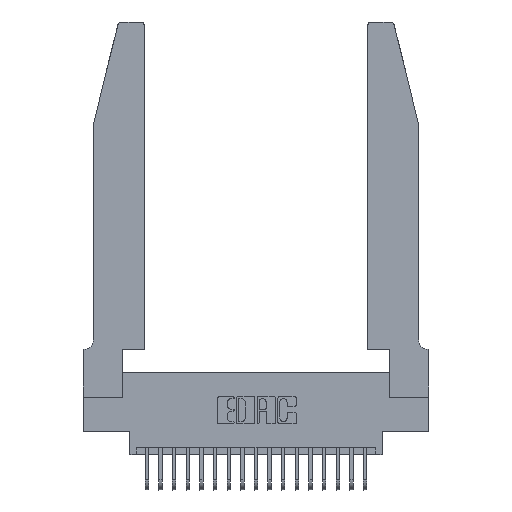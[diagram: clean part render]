
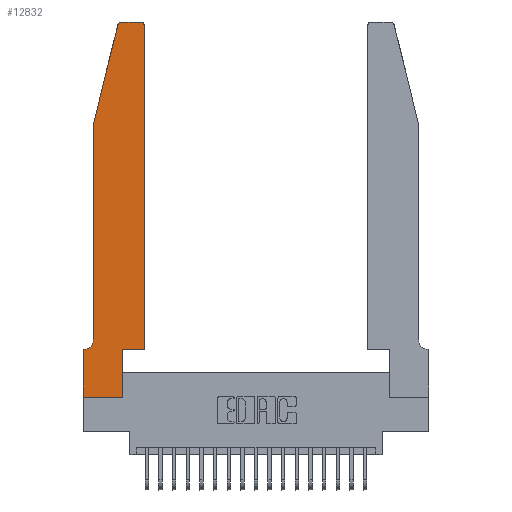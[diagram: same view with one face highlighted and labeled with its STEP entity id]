
A CAD part, top view. The second image highlights one B-rep face of the part: STEP entity #12832.
In plain terms, the highlighted planar face has unit normal (0, 0, 1).
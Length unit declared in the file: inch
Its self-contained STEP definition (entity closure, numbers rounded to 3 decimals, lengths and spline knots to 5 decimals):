
#241 = CARTESIAN_POINT ( 'NONE',  ( 0.2865, 0.35, 0.37 ) ) ;
#877 = EDGE_CURVE ( 'NONE', #9684, #13291, #17296, .T. ) ;
#950 = CARTESIAN_POINT ( 'NONE',  ( 0.4505, 0.35, 0.37 ) ) ;
#2104 = EDGE_CURVE ( 'NONE', #16932, #18440, #22708, .T. ) ;
#2256 = VECTOR ( 'NONE', #17035, 39.37008 ) ;
#2323 = CARTESIAN_POINT ( 'NONE',  ( 0., 0.35, 0.37 ) ) ;
#2464 = CARTESIAN_POINT ( 'NONE',  ( 0.0755, 2., 0.37 ) ) ;
#2515 = CARTESIAN_POINT ( 'NONE',  ( 0.0055, 0.42, 0.37 ) ) ;
#2593 = VERTEX_POINT ( 'NONE', #18004 ) ;
#2752 = AXIS2_PLACEMENT_3D ( 'NONE', #13253, #15020, #4253 ) ;
#3676 = CARTESIAN_POINT ( 'NONE',  ( 0.284, 2.72, 0.37 ) ) ;
#3970 = VERTEX_POINT ( 'NONE', #6643 ) ;
#4253 = DIRECTION ( 'NONE',  ( 1., 0., 0. ) ) ;
#4393 = DIRECTION ( 'NONE',  ( -1., 0., 0. ) ) ;
#4984 = ORIENTED_EDGE ( 'NONE', *, *, #7084, .T. ) ;
#5078 = VERTEX_POINT ( 'NONE', #16766 ) ;
#5187 = CARTESIAN_POINT ( 'NONE',  ( 0.2865, 0., 0.37 ) ) ;
#5199 = VECTOR ( 'NONE', #22372, 39.37008 ) ;
#5392 = CARTESIAN_POINT ( 'NONE',  ( 0.284, 2.75, 0.37 ) ) ;
#5557 = DIRECTION ( 'NONE',  ( 1., 0., 0. ) ) ;
#5711 = EDGE_CURVE ( 'NONE', #18440, #8548, #11969, .T. ) ;
#5781 = LINE ( 'NONE', #20601, #5199 ) ;
#6074 = ORIENTED_EDGE ( 'NONE', *, *, #11623, .T. ) ;
#6567 = VECTOR ( 'NONE', #8561, 39.37008 ) ;
#6643 = CARTESIAN_POINT ( 'NONE',  ( 0.4205, 2.75, 0.37 ) ) ;
#6813 = LINE ( 'NONE', #22697, #11026 ) ;
#6990 = ORIENTED_EDGE ( 'NONE', *, *, #877, .T. ) ;
#7084 = EDGE_CURVE ( 'NONE', #2593, #22466, #12456, .T. ) ;
#7121 = EDGE_CURVE ( 'NONE', #3970, #15149, #11331, .T. ) ;
#7130 = DIRECTION ( 'NONE',  ( 0., 1., 0. ) ) ;
#7306 = DIRECTION ( 'NONE',  ( -1., 0., 0. ) ) ;
#7678 = ORIENTED_EDGE ( 'NONE', *, *, #2104, .T. ) ;
#7838 = EDGE_CURVE ( 'NONE', #16422, #2593, #6813, .T. ) ;
#8370 = CARTESIAN_POINT ( 'NONE',  ( 0.0755, 0.35, 0.37 ) ) ;
#8452 = CARTESIAN_POINT ( 'NONE',  ( 0.4205, 2.72, 0.37 ) ) ;
#8548 = VERTEX_POINT ( 'NONE', #23055 ) ;
#8561 = DIRECTION ( 'NONE',  ( -1., 0., 0. ) ) ;
#8899 = ORIENTED_EDGE ( 'NONE', *, *, #13413, .T. ) ;
#8993 = AXIS2_PLACEMENT_3D ( 'NONE', #3676, #16250, #5557 ) ;
#9684 = VERTEX_POINT ( 'NONE', #2464 ) ;
#9938 = CARTESIAN_POINT ( 'NONE',  ( 0., 0., 0.37 ) ) ;
#10258 = DIRECTION ( 'NONE',  ( 1., 0., 0. ) ) ;
#10673 = CARTESIAN_POINT ( 'NONE',  ( 0.2865, 0.35, 0.37 ) ) ;
#10739 = DIRECTION ( 'NONE',  ( 0., -1., 0. ) ) ;
#11026 = VECTOR ( 'NONE', #13981, 39.37008 ) ;
#11293 = DIRECTION ( 'NONE',  ( 1., 0., 0. ) ) ;
#11321 = CARTESIAN_POINT ( 'NONE',  ( 0.0755, 2., 0.37 ) ) ;
#11331 = LINE ( 'NONE', #13852, #6567 ) ;
#11623 = EDGE_CURVE ( 'NONE', #5078, #9684, #5781, .T. ) ;
#11921 = DIRECTION ( 'NONE',  ( 0., 1., 0. ) ) ;
#11969 = LINE ( 'NONE', #9938, #2256 ) ;
#12070 = EDGE_CURVE ( 'NONE', #19820, #16422, #15271, .T. ) ;
#12185 = LINE ( 'NONE', #20187, #16854 ) ;
#12456 = LINE ( 'NONE', #950, #12991 ) ;
#12832 = ADVANCED_FACE ( 'NONE', ( #22622 ), #21972, .T. ) ;
#12991 = VECTOR ( 'NONE', #11921, 39.37008 ) ;
#13253 = CARTESIAN_POINT ( 'NONE',  ( 0., 0.35, 0.37 ) ) ;
#13291 = VERTEX_POINT ( 'NONE', #18077 ) ;
#13413 = EDGE_CURVE ( 'NONE', #8548, #19820, #12185, .T. ) ;
#13558 = EDGE_LOOP ( 'NONE', ( #17201, #16287, #6074, #6990, #14832, #7678, #20823, #8899, #17856, #15380, #4984, #17040 ) ) ;
#13852 = CARTESIAN_POINT ( 'NONE',  ( 0.2605, 2.75, 0.37 ) ) ;
#13981 = DIRECTION ( 'NONE',  ( 1., 0., 0. ) ) ;
#14418 = CARTESIAN_POINT ( 'NONE',  ( 0.0055, 0.35, 0.37 ) ) ;
#14725 = VECTOR ( 'NONE', #7130, 39.37008 ) ;
#14832 = ORIENTED_EDGE ( 'NONE', *, *, #17916, .T. ) ;
#15020 = DIRECTION ( 'NONE',  ( 0., 0., 1. ) ) ;
#15149 = VERTEX_POINT ( 'NONE', #5392 ) ;
#15150 = DIRECTION ( 'NONE',  ( 0., 0., -1. ) ) ;
#15271 = LINE ( 'NONE', #10673, #14725 ) ;
#15380 = ORIENTED_EDGE ( 'NONE', *, *, #7838, .T. ) ;
#15941 = CIRCLE ( 'NONE', #17163, 0.03 ) ;
#16250 = DIRECTION ( 'NONE',  ( 0., 0., 1. ) ) ;
#16287 = ORIENTED_EDGE ( 'NONE', *, *, #22155, .T. ) ;
#16422 = VERTEX_POINT ( 'NONE', #241 ) ;
#16766 = CARTESIAN_POINT ( 'NONE',  ( 0.25487, 2.72718, 0.37 ) ) ;
#16799 = CIRCLE ( 'NONE', #16855, 0.07 ) ;
#16854 = VECTOR ( 'NONE', #11293, 39.37008 ) ;
#16855 = AXIS2_PLACEMENT_3D ( 'NONE', #2515, #15150, #4393 ) ;
#16932 = VERTEX_POINT ( 'NONE', #14418 ) ;
#17035 = DIRECTION ( 'NONE',  ( 0., -1., 0. ) ) ;
#17040 = ORIENTED_EDGE ( 'NONE', *, *, #18639, .T. ) ;
#17163 = AXIS2_PLACEMENT_3D ( 'NONE', #8452, #20774, #10258 ) ;
#17201 = ORIENTED_EDGE ( 'NONE', *, *, #7121, .T. ) ;
#17296 = LINE ( 'NONE', #11321, #22483 ) ;
#17515 = VECTOR ( 'NONE', #7306, 39.37008 ) ;
#17856 = ORIENTED_EDGE ( 'NONE', *, *, #12070, .T. ) ;
#17916 = EDGE_CURVE ( 'NONE', #13291, #16932, #16799, .T. ) ;
#18004 = CARTESIAN_POINT ( 'NONE',  ( 0.4505, 0.35, 0.37 ) ) ;
#18077 = CARTESIAN_POINT ( 'NONE',  ( 0.0755, 0.42, 0.37 ) ) ;
#18440 = VERTEX_POINT ( 'NONE', #2323 ) ;
#18639 = EDGE_CURVE ( 'NONE', #22466, #3970, #15941, .T. ) ;
#19820 = VERTEX_POINT ( 'NONE', #5187 ) ;
#20018 = CIRCLE ( 'NONE', #8993, 0.03 ) ;
#20187 = CARTESIAN_POINT ( 'NONE',  ( 0., 0., 0.37 ) ) ;
#20502 = CARTESIAN_POINT ( 'NONE',  ( 0.4505, 2.72, 0.37 ) ) ;
#20601 = CARTESIAN_POINT ( 'NONE',  ( 0.0755, 2., 0.37 ) ) ;
#20774 = DIRECTION ( 'NONE',  ( 0., 0., 1. ) ) ;
#20823 = ORIENTED_EDGE ( 'NONE', *, *, #5711, .T. ) ;
#21972 = PLANE ( 'NONE',  #2752 ) ;
#22155 = EDGE_CURVE ( 'NONE', #15149, #5078, #20018, .T. ) ;
#22372 = DIRECTION ( 'NONE',  ( -0.239, -0.971, 0. ) ) ;
#22466 = VERTEX_POINT ( 'NONE', #20502 ) ;
#22483 = VECTOR ( 'NONE', #10739, 39.37008 ) ;
#22622 = FACE_OUTER_BOUND ( 'NONE', #13558, .T. ) ;
#22697 = CARTESIAN_POINT ( 'NONE',  ( 0.4505, 0.35, 0.37 ) ) ;
#22708 = LINE ( 'NONE', #8370, #17515 ) ;
#23055 = CARTESIAN_POINT ( 'NONE',  ( 0., 0., 0.37 ) ) ;
